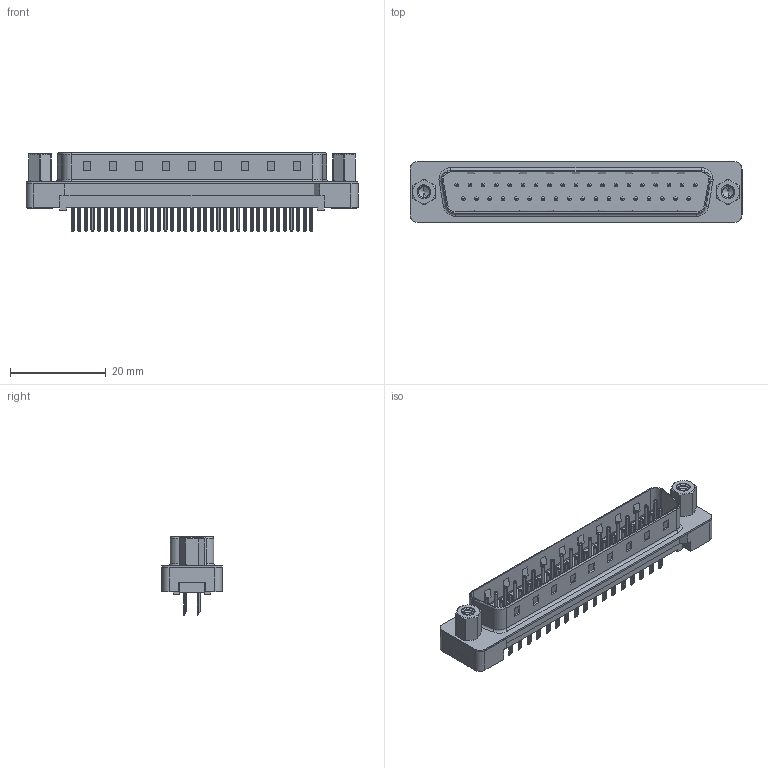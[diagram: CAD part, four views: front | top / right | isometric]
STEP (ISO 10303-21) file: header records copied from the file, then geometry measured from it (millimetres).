
FILE_DESCRIPTION (( 'STEP AP203' ), '1' );
FILE_NAME ('627-037-624-013.STEP', '2020-07-16T02:25:17', ( '' ), ( '' ), 'SwSTEP 2.0', 'SolidWorks 2020', '' );
FILE_SCHEMA (( 'CONFIG_CONTROL_DESIGN' ));
Length unit declared in the file: millimetre
Products named in the file (7): 627 Plastic Body Housing_37 Contacts; 627 PB Contact Row 2_24; 627 PB 4-40 Threaded Rivet; 627 PB Shell_37 Contacts; 627 PB Contact Row 1_24; 627 4-40 Hex Standoff; 627-037-624-013
Assembly tree (43 placements, depth 2):
  627-037-624-013
    627 Plastic Body Housing_37 Contacts
    627 PB Shell_37 Contacts
    627 PB Contact Row 1_24  x19
    627 PB Contact Row 2_24  x18
    627 PB 4-40 Threaded Rivet  x2
    627 4-40 Hex Standoff  x2
Bounding box: 69.32 x 12.6 x 16.3 mm (x, y, z)
Volume: 3432 mm3; surface area: 8244.4 mm2
Topology: 43 solids, 43 shells, 2613 faces, 6962 edges, 4483 vertices
Faces by surface type: plane 1663, cylinder 772, torus 130, cone 30, bspline 18
Entity records: 33955 total; most frequent: CARTESIAN_POINT 9135, ORIENTED_EDGE 4838, DIRECTION 4737, EDGE_CURVE 2419, VECTOR 1701, LINE 1701, VERTEX_POINT 1577, AXIS2_PLACEMENT_3D 1518
